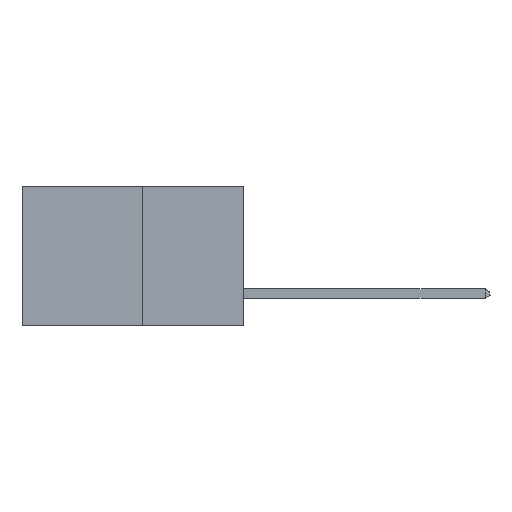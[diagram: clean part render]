
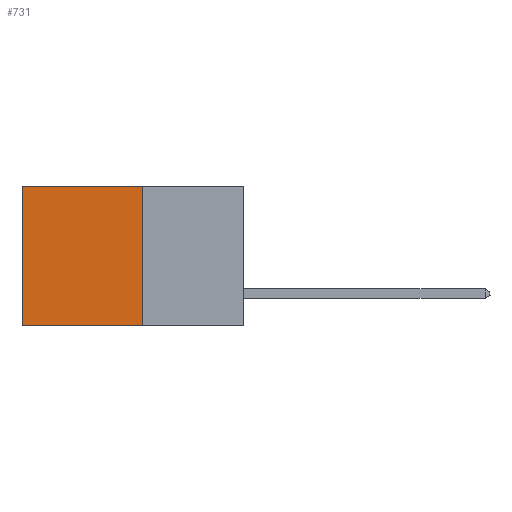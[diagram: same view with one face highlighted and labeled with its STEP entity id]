
A CAD part, left-side view. The second image highlights one B-rep face of the part: STEP entity #731.
In plain terms, the highlighted planar face has unit normal (-1, 0, 0).
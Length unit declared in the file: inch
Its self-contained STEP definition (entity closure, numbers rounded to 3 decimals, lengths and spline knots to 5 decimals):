
#110 = CARTESIAN_POINT ( 'NONE',  ( 0.277, 0.27, -0.37 ) ) ;
#689 = DIRECTION ( 'NONE',  ( 0., 1., 0. ) ) ;
#731 = ADVANCED_FACE ( 'NONE', ( #1971 ), #9699, .F. ) ;
#920 = EDGE_LOOP ( 'NONE', ( #4109, #4199, #4238, #4277 ) ) ;
#1035 = VECTOR ( 'NONE', #2356, 39.37008 ) ;
#1260 = EDGE_CURVE ( 'NONE', #1889, #11631, #5873, .T. ) ;
#1642 = LINE ( 'NONE', #110, #11015 ) ;
#1664 = EDGE_CURVE ( 'NONE', #1889, #11629, #1642, .T. ) ;
#1889 = VERTEX_POINT ( 'NONE', #4264 ) ;
#1971 = FACE_OUTER_BOUND ( 'NONE', #920, .T. ) ;
#2356 = DIRECTION ( 'NONE',  ( 0., 1., 0. ) ) ;
#2630 = CARTESIAN_POINT ( 'NONE',  ( 0.277, 0.59, 0. ) ) ;
#3296 = EDGE_CURVE ( 'NONE', #11631, #6275, #5673, .T. ) ;
#3422 = VECTOR ( 'NONE', #7858, 39.37008 ) ;
#4109 = ORIENTED_EDGE ( 'NONE', *, *, #3296, .T. ) ;
#4199 = ORIENTED_EDGE ( 'NONE', *, *, #9279, .F. ) ;
#4238 = ORIENTED_EDGE ( 'NONE', *, *, #1664, .F. ) ;
#4264 = CARTESIAN_POINT ( 'NONE',  ( 0.277, 0.27, 0. ) ) ;
#4277 = ORIENTED_EDGE ( 'NONE', *, *, #1260, .T. ) ;
#5673 = LINE ( 'NONE', #7695, #3422 ) ;
#5873 = LINE ( 'NONE', #9905, #1035 ) ;
#6275 = VERTEX_POINT ( 'NONE', #8645 ) ;
#6418 = VECTOR ( 'NONE', #689, 39.37008 ) ;
#6420 = CARTESIAN_POINT ( 'NONE',  ( 0.277, 0.27, -0.37 ) ) ;
#6920 = AXIS2_PLACEMENT_3D ( 'NONE', #9077, #9154, #8171 ) ;
#7695 = CARTESIAN_POINT ( 'NONE',  ( 0.277, 0.59, -0.37 ) ) ;
#7858 = DIRECTION ( 'NONE',  ( 0., 0., -1. ) ) ;
#8122 = DIRECTION ( 'NONE',  ( 0., 0., -1. ) ) ;
#8171 = DIRECTION ( 'NONE',  ( 0., 0., -1. ) ) ;
#8200 = CARTESIAN_POINT ( 'NONE',  ( 0.277, 0.27, -0.37 ) ) ;
#8645 = CARTESIAN_POINT ( 'NONE',  ( 0.277, 0.59, -0.37 ) ) ;
#9077 = CARTESIAN_POINT ( 'NONE',  ( 0.277, 0.27, -0.37 ) ) ;
#9154 = DIRECTION ( 'NONE',  ( 1., 0., 0. ) ) ;
#9279 = EDGE_CURVE ( 'NONE', #11629, #6275, #10976, .T. ) ;
#9699 = PLANE ( 'NONE',  #6920 ) ;
#9905 = CARTESIAN_POINT ( 'NONE',  ( 0.277, 0.27, 0. ) ) ;
#10976 = LINE ( 'NONE', #6420, #6418 ) ;
#11015 = VECTOR ( 'NONE', #8122, 39.37008 ) ;
#11629 = VERTEX_POINT ( 'NONE', #8200 ) ;
#11631 = VERTEX_POINT ( 'NONE', #2630 ) ;
